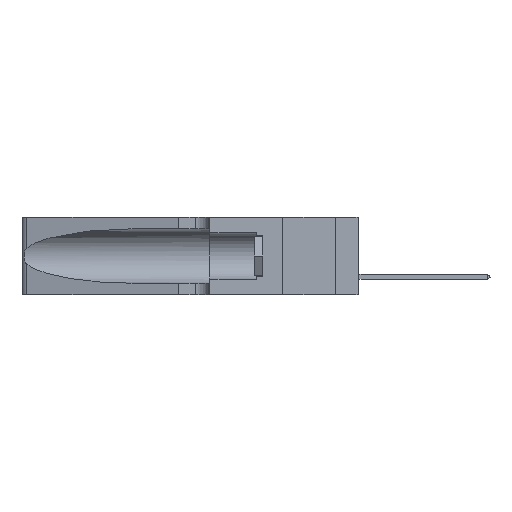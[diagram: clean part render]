
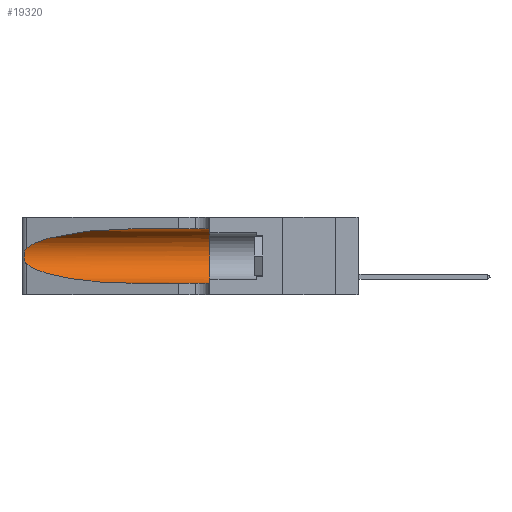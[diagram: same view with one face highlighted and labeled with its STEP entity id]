
A CAD part, left-side view. The second image highlights one B-rep face of the part: STEP entity #19320.
In plain terms, the highlighted cylindrical face has radius 3.308 mm (diameter 6.617 mm), a partial arc.
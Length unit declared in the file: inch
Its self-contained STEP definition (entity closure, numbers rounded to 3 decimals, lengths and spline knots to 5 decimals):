
#164 = EDGE_CURVE ( 'NONE', #10239, #5882, #21079, .T. ) ;
#553 = CARTESIAN_POINT ( 'NONE',  ( 0.2373, 1.15595, 0.08982 ) ) ;
#1658 = DIRECTION ( 'NONE',  ( 0., -1., 0. ) ) ;
#1781 = CARTESIAN_POINT ( 'NONE',  ( 0.25639, 1.23186, 0.15144 ) ) ;
#1951 = DIRECTION ( 'NONE',  ( 0., 0., -1. ) ) ;
#2083 = CARTESIAN_POINT ( 'NONE',  ( 0.25487, 1.22718, 0.14631 ) ) ;
#2331 = CARTESIAN_POINT ( 'NONE',  ( 0.1305, 0.72297, 0.31525 ) ) ;
#4145 = CARTESIAN_POINT ( 'NONE',  ( 0.26018, 1.23835, 0.19895 ) ) ;
#4434 = CARTESIAN_POINT ( 'NONE',  ( 0.1305, 1.61858, 0.05475 ) ) ;
#5216 = CARTESIAN_POINT ( 'NONE',  ( 0.1305, 0.72297, 0.05475 ) ) ;
#5745 = CARTESIAN_POINT ( 'NONE',  ( 0.18966, 0.96281, 0.31525 ) ) ;
#5880 = CARTESIAN_POINT ( 'NONE',  ( 0.1305, 0.72297, 0.05475 ) ) ;
#5882 = VERTEX_POINT ( 'NONE', #12865 ) ;
#6428 = CYLINDRICAL_SURFACE ( 'NONE', #9672, 0.13025 ) ;
#6869 = CARTESIAN_POINT ( 'NONE',  ( 0.18966, 0.96281, 0.05475 ) ) ;
#8217 = ORIENTED_EDGE ( 'NONE', *, *, #164, .F. ) ;
#8297 = CARTESIAN_POINT ( 'NONE',  ( 0.26075, 1.23896, 0.178 ) ) ;
#9672 = AXIS2_PLACEMENT_3D ( 'NONE', #19287, #1658, #1951 ) ;
#9690 = VECTOR ( 'NONE', #11156, 39.37008 ) ;
#9744 = VERTEX_POINT ( 'NONE', #5880 ) ;
#10239 = VERTEX_POINT ( 'NONE', #17905 ) ;
#10685 = CARTESIAN_POINT ( 'NONE',  ( 0.25555, 1.22993, 0.14849 ) ) ;
#10785 = CARTESIAN_POINT ( 'NONE',  ( 0.25487, 1.22718, 0.14631 ) ) ;
#11156 = DIRECTION ( 'NONE',  ( 0., -1., 0. ) ) ;
#11626 = LINE ( 'NONE', #19545, #22580 ) ;
#12457 = CARTESIAN_POINT ( 'NONE',  ( 0.25487, 1.22718, 0.22369 ) ) ;
#12466 = CARTESIAN_POINT ( 'NONE',  ( 0.2373, 1.15595, 0.28018 ) ) ;
#12600 = CARTESIAN_POINT ( 'NONE',  ( 0.1305, 0.35, 0.185 ) ) ;
#12865 = CARTESIAN_POINT ( 'NONE',  ( 0.1305, 0.35, 0.05475 ) ) ;
#12999 = ORIENTED_EDGE ( 'NONE', *, *, #22324, .T. ) ;
#13256 = VERTEX_POINT ( 'NONE', #2083 ) ;
#13962 = ORIENTED_EDGE ( 'NONE', *, *, #18508, .T. ) ;
#14126 =( BOUNDED_CURVE ( )  B_SPLINE_CURVE ( 3, ( #27295, #5745, #12466, #25651 ),
 .UNSPECIFIED., .F., .F. ) 
 B_SPLINE_CURVE_WITH_KNOTS ( ( 4, 4 ),
 ( 1.5708, 2.84003 ),
 .UNSPECIFIED. ) 
 CURVE ( )  GEOMETRIC_REPRESENTATION_ITEM ( )  RATIONAL_B_SPLINE_CURVE ( ( 1., 0.87, 0.87, 1. ) ) 
 REPRESENTATION_ITEM ( '' )  );
#14507 = B_SPLINE_CURVE_WITH_KNOTS ( 'NONE', 3,
 ( #21519, #27918, #17326, #14818, #28008, #4145, #17222, #8297, #23609, #25795, #21708, #1781, #10685, #10785 ),
 .UNSPECIFIED., .F., .F.,
 ( 4, 2, 2, 2, 2, 2, 4 ),
 ( 0., 0.00027, 0.00053, 0.00107, 0.0016, 0.00187, 0.00214 ),
 .UNSPECIFIED. ) ;
#14818 = CARTESIAN_POINT ( 'NONE',  ( 0.25787, 1.23484, 0.2124 ) ) ;
#15538 = LINE ( 'NONE', #4434, #9690 ) ;
#16041 = DIRECTION ( 'NONE',  ( 0., 1., 0. ) ) ;
#17222 = CARTESIAN_POINT ( 'NONE',  ( 0.26075, 1.23896, 0.19203 ) ) ;
#17326 = CARTESIAN_POINT ( 'NONE',  ( 0.25639, 1.23184, 0.21858 ) ) ;
#17340 = AXIS2_PLACEMENT_3D ( 'NONE', #12600, #16041, #22628 ) ;
#17905 = CARTESIAN_POINT ( 'NONE',  ( 0.1305, 0.35, 0.31525 ) ) ;
#18476 = VERTEX_POINT ( 'NONE', #12457 ) ;
#18508 = EDGE_CURVE ( 'NONE', #13256, #9744, #26421, .T. ) ;
#18651 = EDGE_CURVE ( 'NONE', #28210, #10239, #11626, .T. ) ;
#19287 = CARTESIAN_POINT ( 'NONE',  ( 0.1305, 1.61858, 0.185 ) ) ;
#19320 = ADVANCED_FACE ( 'NONE', ( #24222 ), #6428, .F. ) ;
#19545 = CARTESIAN_POINT ( 'NONE',  ( 0.1305, 1.61858, 0.31525 ) ) ;
#19897 = EDGE_CURVE ( 'NONE', #18476, #13256, #14507, .T. ) ;
#20011 = CARTESIAN_POINT ( 'NONE',  ( 0.25487, 1.22718, 0.14631 ) ) ;
#20460 = ORIENTED_EDGE ( 'NONE', *, *, #18651, .F. ) ;
#21079 = CIRCLE ( 'NONE', #17340, 0.13025 ) ;
#21519 = CARTESIAN_POINT ( 'NONE',  ( 0.25487, 1.22718, 0.22369 ) ) ;
#21708 = CARTESIAN_POINT ( 'NONE',  ( 0.25789, 1.23486, 0.15765 ) ) ;
#21821 = ORIENTED_EDGE ( 'NONE', *, *, #19897, .T. ) ;
#22324 = EDGE_CURVE ( 'NONE', #28210, #18476, #14126, .T. ) ;
#22580 = VECTOR ( 'NONE', #25737, 39.37008 ) ;
#22628 = DIRECTION ( 'NONE',  ( 0., 0., 1. ) ) ;
#23215 = ORIENTED_EDGE ( 'NONE', *, *, #25543, .T. ) ;
#23609 = CARTESIAN_POINT ( 'NONE',  ( 0.26017, 1.23833, 0.17102 ) ) ;
#24222 = FACE_OUTER_BOUND ( 'NONE', #25566, .T. ) ;
#25543 = EDGE_CURVE ( 'NONE', #9744, #5882, #15538, .T. ) ;
#25566 = EDGE_LOOP ( 'NONE', ( #12999, #21821, #13962, #23215, #8217, #20460 ) ) ;
#25651 = CARTESIAN_POINT ( 'NONE',  ( 0.25487, 1.22718, 0.22369 ) ) ;
#25737 = DIRECTION ( 'NONE',  ( 0., -1., 0. ) ) ;
#25795 = CARTESIAN_POINT ( 'NONE',  ( 0.25856, 1.23593, 0.16098 ) ) ;
#26421 =( BOUNDED_CURVE ( )  B_SPLINE_CURVE ( 3, ( #20011, #553, #6869, #5216 ),
 .UNSPECIFIED., .F., .F. ) 
 B_SPLINE_CURVE_WITH_KNOTS ( ( 4, 4 ),
 ( 3.44316, 4.71239 ),
 .UNSPECIFIED. ) 
 CURVE ( )  GEOMETRIC_REPRESENTATION_ITEM ( )  RATIONAL_B_SPLINE_CURVE ( ( 1., 0.87, 0.87, 1. ) ) 
 REPRESENTATION_ITEM ( '' )  );
#27295 = CARTESIAN_POINT ( 'NONE',  ( 0.1305, 0.72297, 0.31525 ) ) ;
#27918 = CARTESIAN_POINT ( 'NONE',  ( 0.25555, 1.22994, 0.2215 ) ) ;
#28008 = CARTESIAN_POINT ( 'NONE',  ( 0.25854, 1.2359, 0.20912 ) ) ;
#28210 = VERTEX_POINT ( 'NONE', #2331 ) ;
